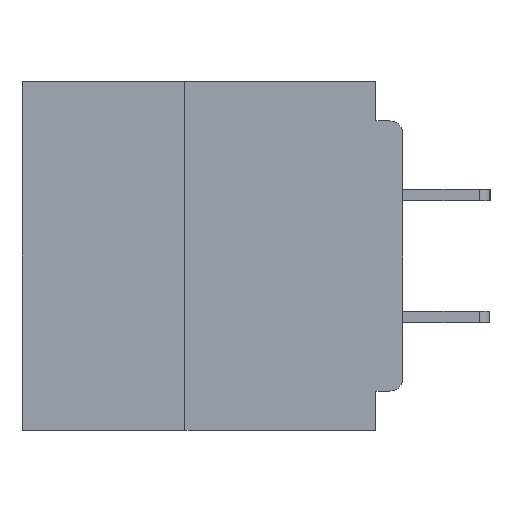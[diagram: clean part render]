
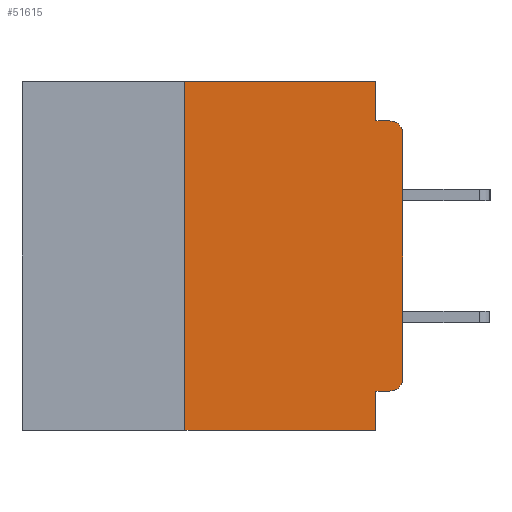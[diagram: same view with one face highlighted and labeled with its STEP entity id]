
A CAD part, left-side view. The second image highlights one B-rep face of the part: STEP entity #51615.
In plain terms, the highlighted planar face has unit normal (-1, 0, 0).
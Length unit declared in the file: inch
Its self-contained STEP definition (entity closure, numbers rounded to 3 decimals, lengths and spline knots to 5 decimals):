
#1012 = EDGE_CURVE ( 'NONE', #9959, #29533, #11208, .T. ) ;
#1641 = CARTESIAN_POINT ( 'NONE',  ( 0., 0.015, -0.34 ) ) ;
#2406 = EDGE_CURVE ( 'NONE', #27486, #57514, #54117, .T. ) ;
#3172 = LINE ( 'NONE', #44909, #50616 ) ;
#3321 = ORIENTED_EDGE ( 'NONE', *, *, #34840, .F. ) ;
#3360 = VERTEX_POINT ( 'NONE', #39552 ) ;
#3507 = EDGE_CURVE ( 'NONE', #59036, #29533, #16073, .T. ) ;
#4345 = ORIENTED_EDGE ( 'NONE', *, *, #3507, .F. ) ;
#4446 = EDGE_CURVE ( 'NONE', #42455, #33556, #36919, .T. ) ;
#5203 = DIRECTION ( 'NONE',  ( 0., -1., 0. ) ) ;
#5417 = CARTESIAN_POINT ( 'NONE',  ( 0., 0., 0. ) ) ;
#5568 = DIRECTION ( 'NONE',  ( 0., -1., 0. ) ) ;
#5735 = LINE ( 'NONE', #33173, #30315 ) ;
#6232 = CARTESIAN_POINT ( 'NONE',  ( 0., 0., -0.355 ) ) ;
#6279 = DIRECTION ( 'NONE',  ( 0., 0., -1. ) ) ;
#7656 = ORIENTED_EDGE ( 'NONE', *, *, #1012, .T. ) ;
#7690 = EDGE_CURVE ( 'NONE', #3360, #27486, #49356, .T. ) ;
#7722 = CIRCLE ( 'NONE', #25305, 0.015 ) ;
#9959 = VERTEX_POINT ( 'NONE', #21081 ) ;
#10553 = DIRECTION ( 'NONE',  ( 0., -1., 0. ) ) ;
#10980 = CIRCLE ( 'NONE', #56566, 0.015 ) ;
#11208 = LINE ( 'NONE', #13381, #55698 ) ;
#12242 = CARTESIAN_POINT ( 'NONE',  ( 0., 0.015, -0.355 ) ) ;
#13381 = CARTESIAN_POINT ( 'NONE',  ( 0., 0.437, -0.4 ) ) ;
#14353 = CARTESIAN_POINT ( 'NONE',  ( 0., 0.437, 0. ) ) ;
#14809 = DIRECTION ( 'NONE',  ( 0., 0., -1. ) ) ;
#14863 = CARTESIAN_POINT ( 'NONE',  ( 0., 0.031, 0. ) ) ;
#16073 = LINE ( 'NONE', #23273, #39102 ) ;
#17140 = CARTESIAN_POINT ( 'NONE',  ( 0., 0., -0.34 ) ) ;
#17377 = DIRECTION ( 'NONE',  ( 0., 0., 1. ) ) ;
#18936 = ORIENTED_EDGE ( 'NONE', *, *, #55225, .T. ) ;
#19018 = DIRECTION ( 'NONE',  ( 1., 0., 0. ) ) ;
#19045 = EDGE_CURVE ( 'NONE', #9959, #3360, #3172, .T. ) ;
#19107 = CARTESIAN_POINT ( 'NONE',  ( 0., 0.031, -0.045 ) ) ;
#21081 = CARTESIAN_POINT ( 'NONE',  ( 0., 0.25, -0.4 ) ) ;
#21757 = ORIENTED_EDGE ( 'NONE', *, *, #7690, .F. ) ;
#22414 = DIRECTION ( 'NONE',  ( 0., 0., -1. ) ) ;
#23273 = CARTESIAN_POINT ( 'NONE',  ( 0., 0.031, -0.4 ) ) ;
#23850 = CARTESIAN_POINT ( 'NONE',  ( 0., 0.015, -0.06 ) ) ;
#23971 = ORIENTED_EDGE ( 'NONE', *, *, #2406, .F. ) ;
#24740 = VECTOR ( 'NONE', #55744, 39.37008 ) ;
#25305 = AXIS2_PLACEMENT_3D ( 'NONE', #23850, #55788, #28522 ) ;
#26794 = CARTESIAN_POINT ( 'NONE',  ( 0., 0.031, 0. ) ) ;
#27486 = VERTEX_POINT ( 'NONE', #26794 ) ;
#28413 = FACE_OUTER_BOUND ( 'NONE', #52221, .T. ) ;
#28522 = DIRECTION ( 'NONE',  ( 0., 0., -1. ) ) ;
#29533 = VERTEX_POINT ( 'NONE', #54479 ) ;
#30315 = VECTOR ( 'NONE', #5568, 39.37008 ) ;
#32455 = ORIENTED_EDGE ( 'NONE', *, *, #19045, .F. ) ;
#32612 = CARTESIAN_POINT ( 'NONE',  ( 0., 0.437, 0. ) ) ;
#33173 = CARTESIAN_POINT ( 'NONE',  ( 0., 0., -0.045 ) ) ;
#33556 = VERTEX_POINT ( 'NONE', #55458 ) ;
#33894 = DIRECTION ( 'NONE',  ( -1., 0., 0. ) ) ;
#34840 = EDGE_CURVE ( 'NONE', #57514, #36692, #5735, .T. ) ;
#35751 = VECTOR ( 'NONE', #5203, 39.37008 ) ;
#36692 = VERTEX_POINT ( 'NONE', #49296 ) ;
#36919 = LINE ( 'NONE', #5417, #24740 ) ;
#39102 = VECTOR ( 'NONE', #22414, 39.37008 ) ;
#39288 = EDGE_CURVE ( 'NONE', #39430, #59036, #46065, .T. ) ;
#39430 = VERTEX_POINT ( 'NONE', #12242 ) ;
#39552 = CARTESIAN_POINT ( 'NONE',  ( 0., 0.25, 0. ) ) ;
#41932 = PLANE ( 'NONE',  #58400 ) ;
#42455 = VERTEX_POINT ( 'NONE', #17140 ) ;
#43219 = VECTOR ( 'NONE', #52216, 39.37008 ) ;
#43461 = VECTOR ( 'NONE', #14809, 39.37008 ) ;
#43519 = ORIENTED_EDGE ( 'NONE', *, *, #4446, .T. ) ;
#44032 = EDGE_CURVE ( 'NONE', #39430, #42455, #10980, .T. ) ;
#44909 = CARTESIAN_POINT ( 'NONE',  ( 0., 0.25, -0.4 ) ) ;
#46065 = LINE ( 'NONE', #6232, #43219 ) ;
#47759 = CARTESIAN_POINT ( 'NONE',  ( 0., 0.031, -0.355 ) ) ;
#49296 = CARTESIAN_POINT ( 'NONE',  ( 0., 0.015, -0.045 ) ) ;
#49356 = LINE ( 'NONE', #32612, #35751 ) ;
#50616 = VECTOR ( 'NONE', #17377, 39.37008 ) ;
#51089 = DIRECTION ( 'NONE',  ( 0., 0., -1. ) ) ;
#51615 = ADVANCED_FACE ( 'NONE', ( #28413 ), #41932, .F. ) ;
#52216 = DIRECTION ( 'NONE',  ( 0., 1., 0. ) ) ;
#52221 = EDGE_LOOP ( 'NONE', ( #43519, #18936, #3321, #23971, #21757, #32455, #7656, #4345, #52847, #54952 ) ) ;
#52847 = ORIENTED_EDGE ( 'NONE', *, *, #39288, .F. ) ;
#54117 = LINE ( 'NONE', #14863, #43461 ) ;
#54479 = CARTESIAN_POINT ( 'NONE',  ( 0., 0.031, -0.4 ) ) ;
#54952 = ORIENTED_EDGE ( 'NONE', *, *, #44032, .T. ) ;
#55225 = EDGE_CURVE ( 'NONE', #33556, #36692, #7722, .T. ) ;
#55458 = CARTESIAN_POINT ( 'NONE',  ( 0., 0., -0.06 ) ) ;
#55698 = VECTOR ( 'NONE', #10553, 39.37008 ) ;
#55744 = DIRECTION ( 'NONE',  ( 0., 0., 1. ) ) ;
#55788 = DIRECTION ( 'NONE',  ( -1., 0., 0. ) ) ;
#56566 = AXIS2_PLACEMENT_3D ( 'NONE', #1641, #33894, #6279 ) ;
#57514 = VERTEX_POINT ( 'NONE', #19107 ) ;
#58400 = AXIS2_PLACEMENT_3D ( 'NONE', #14353, #19018, #51089 ) ;
#59036 = VERTEX_POINT ( 'NONE', #47759 ) ;
